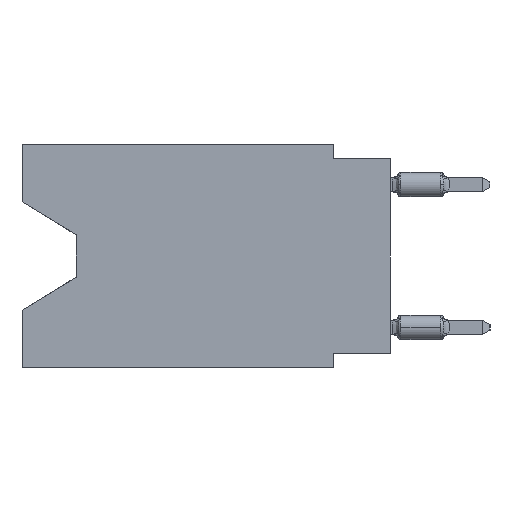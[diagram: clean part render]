
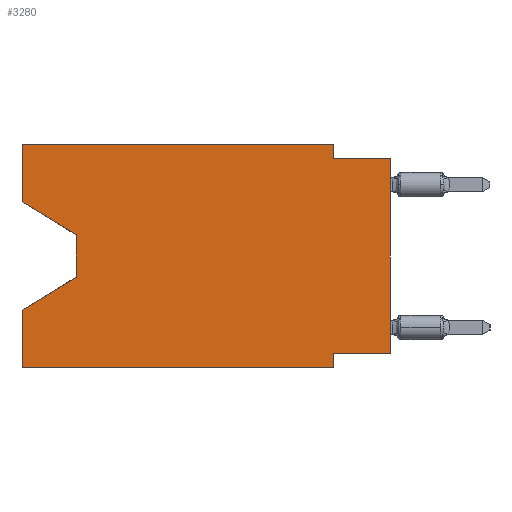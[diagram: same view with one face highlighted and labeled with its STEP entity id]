
A CAD part, left-side view. The second image highlights one B-rep face of the part: STEP entity #3280.
In plain terms, the highlighted planar face has unit normal (-1, 0, 0).
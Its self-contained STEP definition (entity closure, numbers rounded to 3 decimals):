
#2 = CARTESIAN_POINT ( 'NONE',  ( 0., 13.97, -5.893 ) ) ;
#352 = VERTEX_POINT ( 'NONE', #13471 ) ;
#383 = VERTEX_POINT ( 'NONE', #7352 ) ;
#398 = ORIENTED_EDGE ( 'NONE', *, *, #14667, .T. ) ;
#1010 = VECTOR ( 'NONE', #23990, 1000. ) ;
#1811 = CARTESIAN_POINT ( 'NONE',  ( 0., 0., -0.635 ) ) ;
#2565 = DIRECTION ( 'NONE',  ( 0., 0., 1. ) ) ;
#3265 = CARTESIAN_POINT ( 'NONE',  ( 0., 0., 0. ) ) ;
#3280 = ADVANCED_FACE ( 'NONE', ( #3438 ), #9980, .F. ) ;
#3438 = FACE_OUTER_BOUND ( 'NONE', #14163, .T. ) ;
#3461 = VECTOR ( 'NONE', #5642, 1000. ) ;
#3543 = VERTEX_POINT ( 'NONE', #9141 ) ;
#3560 = DIRECTION ( 'NONE',  ( 1., 0., 0. ) ) ;
#3740 = LINE ( 'NONE', #16300, #10028 ) ;
#4202 = DIRECTION ( 'NONE',  ( 0., -1., 0. ) ) ;
#4475 = CARTESIAN_POINT ( 'NONE',  ( 0., 16.383, -2.546 ) ) ;
#4506 = CARTESIAN_POINT ( 'NONE',  ( 0., 13.97, -5.893 ) ) ;
#4966 = CARTESIAN_POINT ( 'NONE',  ( 0., 16.383, 0. ) ) ;
#4971 = VERTEX_POINT ( 'NONE', #4475 ) ;
#5377 = DIRECTION ( 'NONE',  ( 0., -1., 0. ) ) ;
#5642 = DIRECTION ( 'NONE',  ( 0., 1., 0. ) ) ;
#5665 = DIRECTION ( 'NONE',  ( 0., 0., -1. ) ) ;
#6158 = EDGE_CURVE ( 'NONE', #15647, #23223, #6397, .T. ) ;
#6316 = ORIENTED_EDGE ( 'NONE', *, *, #11907, .T. ) ;
#6397 = LINE ( 'NONE', #2, #24412 ) ;
#6769 = EDGE_CURVE ( 'NONE', #3543, #10727, #3740, .T. ) ;
#7352 = CARTESIAN_POINT ( 'NONE',  ( 0., 2.54, -0.635 ) ) ;
#7449 = VERTEX_POINT ( 'NONE', #21875 ) ;
#7930 = DIRECTION ( 'NONE',  ( 0., -0.855, -0.519 ) ) ;
#8692 = ORIENTED_EDGE ( 'NONE', *, *, #6769, .F. ) ;
#9138 = DIRECTION ( 'NONE',  ( 0., -1., 0. ) ) ;
#9141 = CARTESIAN_POINT ( 'NONE',  ( 0., 2.54, -9.271 ) ) ;
#9629 = LINE ( 'NONE', #26300, #1010 ) ;
#9980 = PLANE ( 'NONE',  #16474 ) ;
#10028 = VECTOR ( 'NONE', #12059, 1000. ) ;
#10043 = CARTESIAN_POINT ( 'NONE',  ( 0., 2.54, 0. ) ) ;
#10501 = DIRECTION ( 'NONE',  ( 0., 0.855, -0.519 ) ) ;
#10727 = VERTEX_POINT ( 'NONE', #25010 ) ;
#10914 = LINE ( 'NONE', #11170, #21734 ) ;
#11061 = ORIENTED_EDGE ( 'NONE', *, *, #12288, .T. ) ;
#11170 = CARTESIAN_POINT ( 'NONE',  ( 0., 0., -0.635 ) ) ;
#11792 = LINE ( 'NONE', #26014, #3461 ) ;
#11907 = EDGE_CURVE ( 'NONE', #4971, #352, #18866, .T. ) ;
#11962 = EDGE_CURVE ( 'NONE', #383, #15494, #10914, .T. ) ;
#12059 = DIRECTION ( 'NONE',  ( 0., 0., -1. ) ) ;
#12236 = ORIENTED_EDGE ( 'NONE', *, *, #6158, .T. ) ;
#12288 = EDGE_CURVE ( 'NONE', #17252, #10727, #14448, .T. ) ;
#12385 = CARTESIAN_POINT ( 'NONE',  ( 0., 16.383, 0. ) ) ;
#12440 = EDGE_CURVE ( 'NONE', #17252, #23223, #17290, .T. ) ;
#12687 = ORIENTED_EDGE ( 'NONE', *, *, #22649, .T. ) ;
#12727 = LINE ( 'NONE', #19029, #12736 ) ;
#12736 = VECTOR ( 'NONE', #21084, 1000. ) ;
#12743 = VERTEX_POINT ( 'NONE', #10043 ) ;
#12959 = VECTOR ( 'NONE', #20195, 1000. ) ;
#12963 = EDGE_CURVE ( 'NONE', #22358, #12743, #19731, .T. ) ;
#13471 = CARTESIAN_POINT ( 'NONE',  ( 0., 13.97, -4.013 ) ) ;
#13790 = DIRECTION ( 'NONE',  ( 0., 0., -1. ) ) ;
#13868 = VECTOR ( 'NONE', #5377, 1000. ) ;
#14163 = EDGE_LOOP ( 'NONE', ( #6316, #12687, #12236, #24782, #11061, #8692, #21555, #398, #19910, #22664, #24755, #23198 ) ) ;
#14305 = CARTESIAN_POINT ( 'NONE',  ( 0., 16.383, -9.906 ) ) ;
#14448 = LINE ( 'NONE', #14305, #15592 ) ;
#14619 = CARTESIAN_POINT ( 'NONE',  ( 0., 16.383, -2.546 ) ) ;
#14667 = EDGE_CURVE ( 'NONE', #7449, #15494, #19925, .T. ) ;
#15494 = VERTEX_POINT ( 'NONE', #1811 ) ;
#15592 = VECTOR ( 'NONE', #4202, 1000. ) ;
#15647 = VERTEX_POINT ( 'NONE', #4506 ) ;
#15976 = CARTESIAN_POINT ( 'NONE',  ( 0., 16.383, 0. ) ) ;
#16300 = CARTESIAN_POINT ( 'NONE',  ( 0., 2.54, -9.906 ) ) ;
#16474 = AXIS2_PLACEMENT_3D ( 'NONE', #15976, #3560, #13790 ) ;
#16893 = CARTESIAN_POINT ( 'NONE',  ( 0., 16.383, 0. ) ) ;
#17252 = VERTEX_POINT ( 'NONE', #26621 ) ;
#17290 = LINE ( 'NONE', #16893, #24344 ) ;
#17697 = CARTESIAN_POINT ( 'NONE',  ( 0., 2.54, 0. ) ) ;
#18082 = EDGE_CURVE ( 'NONE', #7449, #3543, #11792, .T. ) ;
#18866 = LINE ( 'NONE', #14619, #23053 ) ;
#19029 = CARTESIAN_POINT ( 'NONE',  ( 0., 16.383, 0. ) ) ;
#19731 = LINE ( 'NONE', #4966, #13868 ) ;
#19910 = ORIENTED_EDGE ( 'NONE', *, *, #11962, .F. ) ;
#19925 = LINE ( 'NONE', #3265, #12959 ) ;
#20195 = DIRECTION ( 'NONE',  ( 0., 0., 1. ) ) ;
#21084 = DIRECTION ( 'NONE',  ( 0., 0., 1. ) ) ;
#21555 = ORIENTED_EDGE ( 'NONE', *, *, #18082, .F. ) ;
#21734 = VECTOR ( 'NONE', #9138, 1000. ) ;
#21875 = CARTESIAN_POINT ( 'NONE',  ( 0., 0., -9.271 ) ) ;
#22358 = VERTEX_POINT ( 'NONE', #12385 ) ;
#22649 = EDGE_CURVE ( 'NONE', #352, #15647, #9629, .T. ) ;
#22664 = ORIENTED_EDGE ( 'NONE', *, *, #25052, .F. ) ;
#23053 = VECTOR ( 'NONE', #7930, 1000. ) ;
#23198 = ORIENTED_EDGE ( 'NONE', *, *, #25677, .F. ) ;
#23223 = VERTEX_POINT ( 'NONE', #25142 ) ;
#23990 = DIRECTION ( 'NONE',  ( 0., 0., -1. ) ) ;
#24344 = VECTOR ( 'NONE', #2565, 1000. ) ;
#24397 = LINE ( 'NONE', #17697, #26728 ) ;
#24412 = VECTOR ( 'NONE', #10501, 1000. ) ;
#24755 = ORIENTED_EDGE ( 'NONE', *, *, #12963, .F. ) ;
#24782 = ORIENTED_EDGE ( 'NONE', *, *, #12440, .F. ) ;
#25010 = CARTESIAN_POINT ( 'NONE',  ( 0., 2.54, -9.906 ) ) ;
#25052 = EDGE_CURVE ( 'NONE', #12743, #383, #24397, .T. ) ;
#25142 = CARTESIAN_POINT ( 'NONE',  ( 0., 16.383, -7.36 ) ) ;
#25677 = EDGE_CURVE ( 'NONE', #4971, #22358, #12727, .T. ) ;
#26014 = CARTESIAN_POINT ( 'NONE',  ( 0., 0., -9.271 ) ) ;
#26300 = CARTESIAN_POINT ( 'NONE',  ( 0., 13.97, -4.013 ) ) ;
#26621 = CARTESIAN_POINT ( 'NONE',  ( 0., 16.383, -9.906 ) ) ;
#26728 = VECTOR ( 'NONE', #5665, 1000. ) ;
